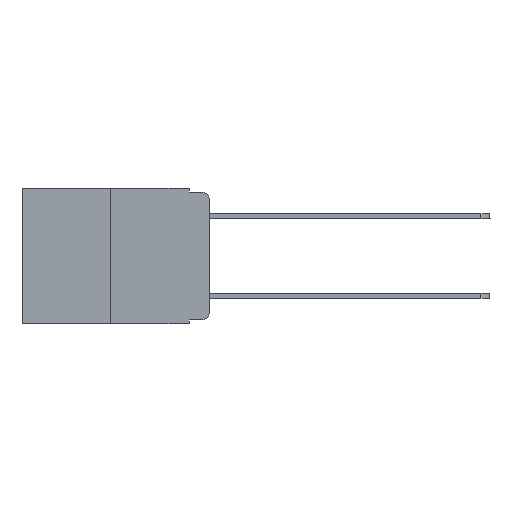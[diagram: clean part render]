
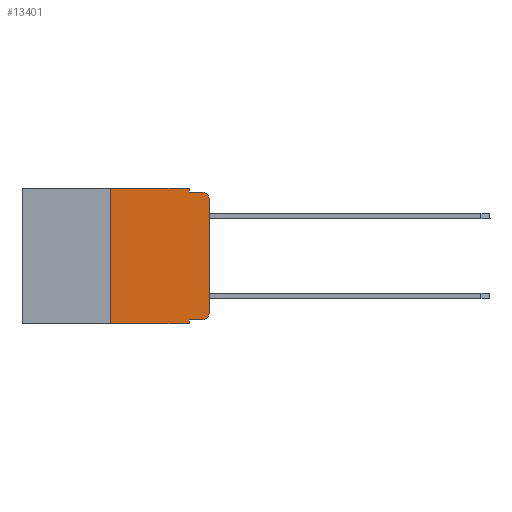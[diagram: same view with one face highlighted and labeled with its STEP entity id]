
A CAD part, left-side view. The second image highlights one B-rep face of the part: STEP entity #13401.
In plain terms, the highlighted planar face has unit normal (-1, 0, 0).
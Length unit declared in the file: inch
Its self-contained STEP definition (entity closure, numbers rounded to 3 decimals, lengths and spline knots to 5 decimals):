
#1896 = CARTESIAN_POINT ( 'NONE',  ( 0., 0., -0.03 ) ) ;
#1938 = ORIENTED_EDGE ( 'NONE', *, *, #14232, .T. ) ;
#2097 = LINE ( 'NONE', #19148, #13251 ) ;
#2163 = CARTESIAN_POINT ( 'NONE',  ( 0., 0.473, 0. ) ) ;
#2527 = LINE ( 'NONE', #11920, #11372 ) ;
#2767 = LINE ( 'NONE', #10364, #16061 ) ;
#3705 = LINE ( 'NONE', #15589, #10301 ) ;
#3788 = VERTEX_POINT ( 'NONE', #6593 ) ;
#4317 = EDGE_CURVE ( 'NONE', #21333, #20326, #14471, .T. ) ;
#4537 = VECTOR ( 'NONE', #13367, 39.37008 ) ;
#4641 = ORIENTED_EDGE ( 'NONE', *, *, #4317, .T. ) ;
#5194 = CARTESIAN_POINT ( 'NONE',  ( 0., 0., 0. ) ) ;
#5245 = CIRCLE ( 'NONE', #20881, 0.02 ) ;
#5304 = ORIENTED_EDGE ( 'NONE', *, *, #23427, .F. ) ;
#5852 = CARTESIAN_POINT ( 'NONE',  ( 0., 0.02, -0.333 ) ) ;
#6593 = CARTESIAN_POINT ( 'NONE',  ( 0., 0.051, -0.01 ) ) ;
#7233 = ORIENTED_EDGE ( 'NONE', *, *, #24369, .F. ) ;
#7758 = EDGE_CURVE ( 'NONE', #15398, #13828, #2097, .T. ) ;
#7786 = AXIS2_PLACEMENT_3D ( 'NONE', #9051, #16700, #12698 ) ;
#8263 = PLANE ( 'NONE',  #20681 ) ;
#8351 = EDGE_CURVE ( 'NONE', #8421, #15932, #2767, .T. ) ;
#8382 = DIRECTION ( 'NONE',  ( 0., 0., -1. ) ) ;
#8421 = VERTEX_POINT ( 'NONE', #20782 ) ;
#8728 = CARTESIAN_POINT ( 'NONE',  ( 0., 0.25, 0. ) ) ;
#9051 = CARTESIAN_POINT ( 'NONE',  ( 0., 0.02, -0.313 ) ) ;
#9208 = VECTOR ( 'NONE', #21992, 39.37008 ) ;
#9266 = DIRECTION ( 'NONE',  ( -1., 0., 0. ) ) ;
#9873 = VECTOR ( 'NONE', #12119, 39.37008 ) ;
#9894 = DIRECTION ( 'NONE',  ( 1., 0., 0. ) ) ;
#9999 = CARTESIAN_POINT ( 'NONE',  ( 0., 0., -0.313 ) ) ;
#10301 = VECTOR ( 'NONE', #11449, 39.37008 ) ;
#10364 = CARTESIAN_POINT ( 'NONE',  ( 0., 0.051, -0.333 ) ) ;
#10759 = CARTESIAN_POINT ( 'NONE',  ( 0., 0.02, -0.01 ) ) ;
#11167 = VERTEX_POINT ( 'NONE', #15067 ) ;
#11372 = VECTOR ( 'NONE', #19809, 39.37008 ) ;
#11449 = DIRECTION ( 'NONE',  ( 0., -1., 0. ) ) ;
#11744 = CARTESIAN_POINT ( 'NONE',  ( 0., 0.051, -0.01 ) ) ;
#11815 = CARTESIAN_POINT ( 'NONE',  ( 0., 0.25, -0.343 ) ) ;
#11918 = EDGE_CURVE ( 'NONE', #8421, #11167, #12937, .T. ) ;
#11920 = CARTESIAN_POINT ( 'NONE',  ( 0., 0.25, 0. ) ) ;
#12119 = DIRECTION ( 'NONE',  ( 0., -1., 0. ) ) ;
#12698 = DIRECTION ( 'NONE',  ( 0., 0., -1. ) ) ;
#12856 = ORIENTED_EDGE ( 'NONE', *, *, #7758, .F. ) ;
#12937 = LINE ( 'NONE', #18714, #21819 ) ;
#13251 = VECTOR ( 'NONE', #19258, 39.37008 ) ;
#13367 = DIRECTION ( 'NONE',  ( 0., 0., -1. ) ) ;
#13401 = ADVANCED_FACE ( 'NONE', ( #21423 ), #8263, .F. ) ;
#13640 = LINE ( 'NONE', #11744, #9873 ) ;
#13825 = EDGE_CURVE ( 'NONE', #3788, #24563, #13640, .T. ) ;
#13828 = VERTEX_POINT ( 'NONE', #21163 ) ;
#14232 = EDGE_CURVE ( 'NONE', #14296, #11167, #3705, .T. ) ;
#14296 = VERTEX_POINT ( 'NONE', #11815 ) ;
#14471 = LINE ( 'NONE', #5194, #9208 ) ;
#14981 = CIRCLE ( 'NONE', #7786, 0.02 ) ;
#15067 = CARTESIAN_POINT ( 'NONE',  ( 0., 0.051, -0.343 ) ) ;
#15252 = LINE ( 'NONE', #22891, #4537 ) ;
#15398 = VERTEX_POINT ( 'NONE', #8728 ) ;
#15589 = CARTESIAN_POINT ( 'NONE',  ( 0., 0.473, -0.343 ) ) ;
#15932 = VERTEX_POINT ( 'NONE', #5852 ) ;
#16061 = VECTOR ( 'NONE', #23793, 39.37008 ) ;
#16543 = DIRECTION ( 'NONE',  ( 0., 0., -1. ) ) ;
#16700 = DIRECTION ( 'NONE',  ( -1., 0., 0. ) ) ;
#16804 = ORIENTED_EDGE ( 'NONE', *, *, #24022, .T. ) ;
#17112 = EDGE_CURVE ( 'NONE', #20326, #24563, #5245, .T. ) ;
#17395 = DIRECTION ( 'NONE',  ( 0., 0., -1. ) ) ;
#17798 = ORIENTED_EDGE ( 'NONE', *, *, #17112, .T. ) ;
#18714 = CARTESIAN_POINT ( 'NONE',  ( 0., 0.051, 0. ) ) ;
#19148 = CARTESIAN_POINT ( 'NONE',  ( 0., 0.473, 0. ) ) ;
#19258 = DIRECTION ( 'NONE',  ( 0., -1., 0. ) ) ;
#19809 = DIRECTION ( 'NONE',  ( 0., 0., 1. ) ) ;
#20326 = VERTEX_POINT ( 'NONE', #1896 ) ;
#20557 = CARTESIAN_POINT ( 'NONE',  ( 0., 0.02, -0.03 ) ) ;
#20681 = AXIS2_PLACEMENT_3D ( 'NONE', #2163, #9894, #8382 ) ;
#20782 = CARTESIAN_POINT ( 'NONE',  ( 0., 0.051, -0.333 ) ) ;
#20881 = AXIS2_PLACEMENT_3D ( 'NONE', #20557, #9266, #16543 ) ;
#21163 = CARTESIAN_POINT ( 'NONE',  ( 0., 0.051, 0. ) ) ;
#21333 = VERTEX_POINT ( 'NONE', #9999 ) ;
#21423 = FACE_OUTER_BOUND ( 'NONE', #23942, .T. ) ;
#21806 = ORIENTED_EDGE ( 'NONE', *, *, #11918, .F. ) ;
#21819 = VECTOR ( 'NONE', #17395, 39.37008 ) ;
#21992 = DIRECTION ( 'NONE',  ( 0., 0., 1. ) ) ;
#22891 = CARTESIAN_POINT ( 'NONE',  ( 0., 0.051, 0. ) ) ;
#23427 = EDGE_CURVE ( 'NONE', #13828, #3788, #15252, .T. ) ;
#23728 = ORIENTED_EDGE ( 'NONE', *, *, #13825, .F. ) ;
#23793 = DIRECTION ( 'NONE',  ( 0., -1., 0. ) ) ;
#23942 = EDGE_LOOP ( 'NONE', ( #4641, #17798, #23728, #5304, #12856, #7233, #1938, #21806, #24645, #16804 ) ) ;
#24022 = EDGE_CURVE ( 'NONE', #15932, #21333, #14981, .T. ) ;
#24369 = EDGE_CURVE ( 'NONE', #14296, #15398, #2527, .T. ) ;
#24563 = VERTEX_POINT ( 'NONE', #10759 ) ;
#24645 = ORIENTED_EDGE ( 'NONE', *, *, #8351, .T. ) ;
